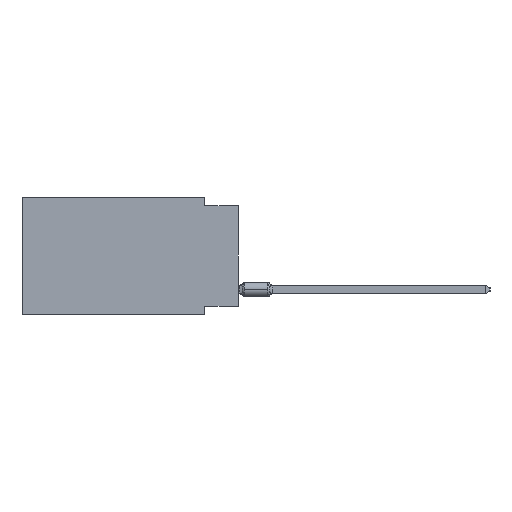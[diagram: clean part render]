
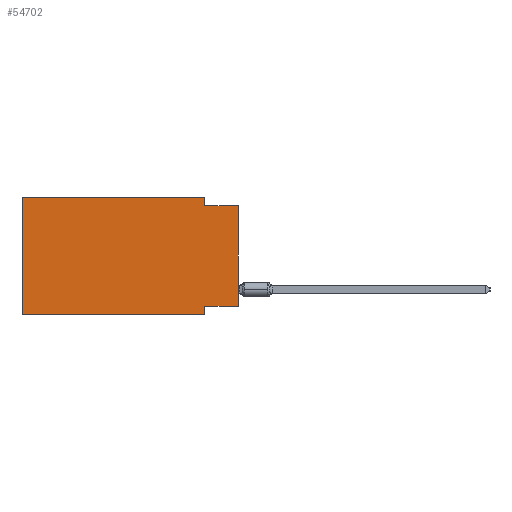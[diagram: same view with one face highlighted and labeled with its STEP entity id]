
A CAD part, left-side view. The second image highlights one B-rep face of the part: STEP entity #54702.
In plain terms, the highlighted planar face has unit normal (-1, 0, 0).
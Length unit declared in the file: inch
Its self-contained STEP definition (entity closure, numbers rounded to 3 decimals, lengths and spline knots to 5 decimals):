
#3284 = EDGE_CURVE ( 'NONE', #40781, #13178, #36035, .T. ) ;
#4509 = VERTEX_POINT ( 'NONE', #27668 ) ;
#4626 = LINE ( 'NONE', #37591, #19163 ) ;
#4631 = CARTESIAN_POINT ( 'NONE',  ( 0., 0.645, 0. ) ) ;
#4861 = EDGE_LOOP ( 'NONE', ( #32035, #8137, #23888, #13497, #30531, #9474, #25599, #44528 ) ) ;
#6693 = CARTESIAN_POINT ( 'NONE',  ( 0., 0.1, -0.025 ) ) ;
#6956 = LINE ( 'NONE', #10340, #18182 ) ;
#7067 = VECTOR ( 'NONE', #10820, 39.37008 ) ;
#7436 = EDGE_CURVE ( 'NONE', #45702, #28181, #50716, .T. ) ;
#8137 = ORIENTED_EDGE ( 'NONE', *, *, #23409, .F. ) ;
#9086 = VECTOR ( 'NONE', #37130, 39.37008 ) ;
#9474 = ORIENTED_EDGE ( 'NONE', *, *, #20235, .T. ) ;
#10340 = CARTESIAN_POINT ( 'NONE',  ( 0., 0.645, -0.35 ) ) ;
#10820 = DIRECTION ( 'NONE',  ( 0., -1., 0. ) ) ;
#12453 = CARTESIAN_POINT ( 'NONE',  ( 0., 0., -0.025 ) ) ;
#12655 = VERTEX_POINT ( 'NONE', #6693 ) ;
#13178 = VERTEX_POINT ( 'NONE', #12453 ) ;
#13497 = ORIENTED_EDGE ( 'NONE', *, *, #17453, .F. ) ;
#14488 = VECTOR ( 'NONE', #25965, 39.37008 ) ;
#14819 = CARTESIAN_POINT ( 'NONE',  ( 0., 0., 0. ) ) ;
#17161 = CARTESIAN_POINT ( 'NONE',  ( 0., 0.645, 0. ) ) ;
#17453 = EDGE_CURVE ( 'NONE', #28181, #22421, #55141, .T. ) ;
#18182 = VECTOR ( 'NONE', #19296, 39.37008 ) ;
#18951 = CARTESIAN_POINT ( 'NONE',  ( 0., 0.645, 0. ) ) ;
#19163 = VECTOR ( 'NONE', #51273, 39.37008 ) ;
#19296 = DIRECTION ( 'NONE',  ( 0., -1., 0. ) ) ;
#20235 = EDGE_CURVE ( 'NONE', #45702, #4509, #6956, .T. ) ;
#20479 = CARTESIAN_POINT ( 'NONE',  ( 0., 0., -0.325 ) ) ;
#20781 = CARTESIAN_POINT ( 'NONE',  ( 0., 0.645, -0.35 ) ) ;
#22421 = VERTEX_POINT ( 'NONE', #39525 ) ;
#23409 = EDGE_CURVE ( 'NONE', #12655, #13178, #41232, .T. ) ;
#23888 = ORIENTED_EDGE ( 'NONE', *, *, #35057, .F. ) ;
#23990 = FACE_OUTER_BOUND ( 'NONE', #4861, .T. ) ;
#25166 = VECTOR ( 'NONE', #46135, 39.37008 ) ;
#25599 = ORIENTED_EDGE ( 'NONE', *, *, #37137, .F. ) ;
#25965 = DIRECTION ( 'NONE',  ( 0., 0., -1. ) ) ;
#27021 = CARTESIAN_POINT ( 'NONE',  ( 0., 0.1, 0. ) ) ;
#27668 = CARTESIAN_POINT ( 'NONE',  ( 0., 0.1, -0.35 ) ) ;
#28181 = VERTEX_POINT ( 'NONE', #18951 ) ;
#28670 = CARTESIAN_POINT ( 'NONE',  ( 0., 0.1, -0.325 ) ) ;
#30047 = DIRECTION ( 'NONE',  ( 0., 0., 1. ) ) ;
#30531 = ORIENTED_EDGE ( 'NONE', *, *, #7436, .F. ) ;
#32035 = ORIENTED_EDGE ( 'NONE', *, *, #3284, .T. ) ;
#32378 = PLANE ( 'NONE',  #51948 ) ;
#34423 = EDGE_CURVE ( 'NONE', #40781, #36986, #46412, .T. ) ;
#34473 = DIRECTION ( 'NONE',  ( 0., -1., 0. ) ) ;
#35057 = EDGE_CURVE ( 'NONE', #22421, #12655, #50819, .T. ) ;
#35948 = VECTOR ( 'NONE', #34473, 39.37008 ) ;
#36035 = LINE ( 'NONE', #14819, #9086 ) ;
#36986 = VERTEX_POINT ( 'NONE', #28670 ) ;
#37130 = DIRECTION ( 'NONE',  ( 0., 0., 1. ) ) ;
#37137 = EDGE_CURVE ( 'NONE', #36986, #4509, #4626, .T. ) ;
#37591 = CARTESIAN_POINT ( 'NONE',  ( 0., 0.1, -0.35 ) ) ;
#39525 = CARTESIAN_POINT ( 'NONE',  ( 0., 0.1, 0. ) ) ;
#40781 = VERTEX_POINT ( 'NONE', #54371 ) ;
#40985 = DIRECTION ( 'NONE',  ( 1., 0., 0. ) ) ;
#41232 = LINE ( 'NONE', #53267, #7067 ) ;
#44528 = ORIENTED_EDGE ( 'NONE', *, *, #34423, .F. ) ;
#45188 = DIRECTION ( 'NONE',  ( 0., 0., -1. ) ) ;
#45702 = VERTEX_POINT ( 'NONE', #20781 ) ;
#46135 = DIRECTION ( 'NONE',  ( 0., 1., 0. ) ) ;
#46412 = LINE ( 'NONE', #20479, #25166 ) ;
#49393 = CARTESIAN_POINT ( 'NONE',  ( 0., 0.645, 0. ) ) ;
#50716 = LINE ( 'NONE', #4631, #55224 ) ;
#50819 = LINE ( 'NONE', #27021, #14488 ) ;
#51273 = DIRECTION ( 'NONE',  ( 0., 0., -1. ) ) ;
#51948 = AXIS2_PLACEMENT_3D ( 'NONE', #49393, #40985, #45188 ) ;
#53267 = CARTESIAN_POINT ( 'NONE',  ( 0., 0., -0.025 ) ) ;
#54371 = CARTESIAN_POINT ( 'NONE',  ( 0., 0., -0.325 ) ) ;
#54702 = ADVANCED_FACE ( 'NONE', ( #23990 ), #32378, .F. ) ;
#55141 = LINE ( 'NONE', #17161, #35948 ) ;
#55224 = VECTOR ( 'NONE', #30047, 39.37008 ) ;
